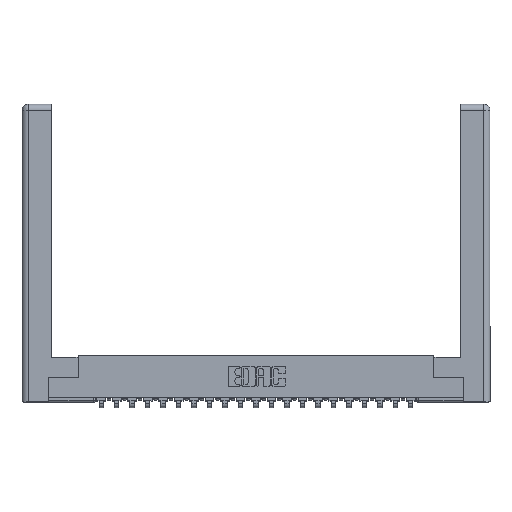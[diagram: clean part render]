
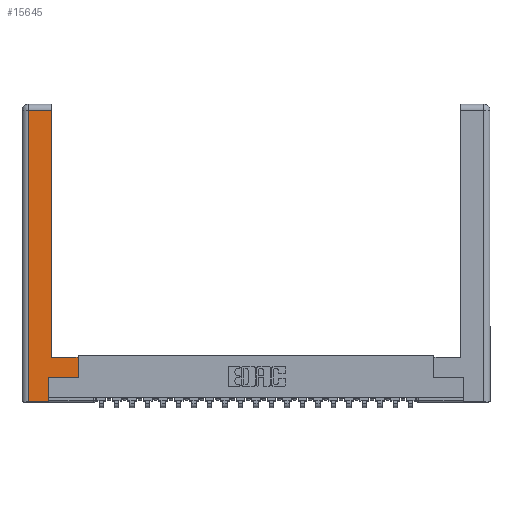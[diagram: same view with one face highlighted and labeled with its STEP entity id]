
A CAD part, top view. The second image highlights one B-rep face of the part: STEP entity #15645.
In plain terms, the highlighted planar face has unit normal (0, 0, 1).
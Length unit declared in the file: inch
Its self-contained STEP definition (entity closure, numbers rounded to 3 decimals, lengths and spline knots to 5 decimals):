
#306 = PLANE ( 'NONE',  #10145 ) ;
#809 = CARTESIAN_POINT ( 'NONE',  ( 0.295, 0.45, 0. ) ) ;
#877 = EDGE_CURVE ( 'NONE', #16083, #6153, #20618, .T. ) ;
#1115 = CARTESIAN_POINT ( 'NONE',  ( 0.265, 0., 0. ) ) ;
#1263 = ORIENTED_EDGE ( 'NONE', *, *, #13208, .T. ) ;
#1589 = VECTOR ( 'NONE', #19263, 39.37008 ) ;
#1649 = DIRECTION ( 'NONE',  ( 0., -1., 0. ) ) ;
#1656 = ORIENTED_EDGE ( 'NONE', *, *, #18970, .T. ) ;
#2031 = DIRECTION ( 'NONE',  ( -1., 0., 0. ) ) ;
#2057 = LINE ( 'NONE', #20446, #7541 ) ;
#2531 = ORIENTED_EDGE ( 'NONE', *, *, #13943, .T. ) ;
#2829 = LINE ( 'NONE', #1115, #1589 ) ;
#3650 = VERTEX_POINT ( 'NONE', #5099 ) ;
#3750 = ORIENTED_EDGE ( 'NONE', *, *, #877, .T. ) ;
#4056 = ORIENTED_EDGE ( 'NONE', *, *, #12929, .T. ) ;
#4154 = CARTESIAN_POINT ( 'NONE',  ( 0.265, 0.245, 0. ) ) ;
#5099 = CARTESIAN_POINT ( 'NONE',  ( 0.265, 0., 0. ) ) ;
#6027 = CARTESIAN_POINT ( 'NONE',  ( 0.565, 0.45, 0. ) ) ;
#6153 = VERTEX_POINT ( 'NONE', #6720 ) ;
#6720 = CARTESIAN_POINT ( 'NONE',  ( 0.295, 2.94, 0. ) ) ;
#7017 = ORIENTED_EDGE ( 'NONE', *, *, #14044, .T. ) ;
#7489 = VERTEX_POINT ( 'NONE', #21320 ) ;
#7541 = VECTOR ( 'NONE', #19099, 39.37008 ) ;
#8153 = VERTEX_POINT ( 'NONE', #20661 ) ;
#8188 = LINE ( 'NONE', #22556, #16856 ) ;
#8681 = VECTOR ( 'NONE', #20383, 39.37008 ) ;
#8954 = CARTESIAN_POINT ( 'NONE',  ( 0.0615, 0., 0. ) ) ;
#8990 = ORIENTED_EDGE ( 'NONE', *, *, #10652, .T. ) ;
#9011 = CARTESIAN_POINT ( 'NONE',  ( 0.0615, 0., 0. ) ) ;
#9062 = DIRECTION ( 'NONE',  ( 0., 1., 0. ) ) ;
#10145 = AXIS2_PLACEMENT_3D ( 'NONE', #20664, #11296, #2031 ) ;
#10652 = EDGE_CURVE ( 'NONE', #18060, #3650, #2829, .T. ) ;
#11296 = DIRECTION ( 'NONE',  ( 0., 0., -1. ) ) ;
#12262 = VERTEX_POINT ( 'NONE', #4154 ) ;
#12383 = ORIENTED_EDGE ( 'NONE', *, *, #21608, .T. ) ;
#12608 = VECTOR ( 'NONE', #20359, 39.37008 ) ;
#12929 = EDGE_CURVE ( 'NONE', #3650, #12262, #22329, .T. ) ;
#12940 = CARTESIAN_POINT ( 'NONE',  ( 0.565, 0.245, 0. ) ) ;
#13076 = CARTESIAN_POINT ( 'NONE',  ( 0.265, 0.245, 0. ) ) ;
#13208 = EDGE_CURVE ( 'NONE', #6153, #7489, #8188, .T. ) ;
#13326 = CARTESIAN_POINT ( 'NONE',  ( 0.295, 0.45, 0. ) ) ;
#13896 = VECTOR ( 'NONE', #9062, 39.37008 ) ;
#13943 = EDGE_CURVE ( 'NONE', #21923, #16083, #15541, .T. ) ;
#14044 = EDGE_CURVE ( 'NONE', #8153, #21923, #2057, .T. ) ;
#15541 = LINE ( 'NONE', #809, #17268 ) ;
#15616 = DIRECTION ( 'NONE',  ( -1., 0., 0. ) ) ;
#15645 = ADVANCED_FACE ( 'NONE', ( #22366 ), #306, .F. ) ;
#15664 = DIRECTION ( 'NONE',  ( -1., 0., 0. ) ) ;
#16083 = VERTEX_POINT ( 'NONE', #13326 ) ;
#16856 = VECTOR ( 'NONE', #15616, 39.37008 ) ;
#17268 = VECTOR ( 'NONE', #15664, 39.37008 ) ;
#17886 = EDGE_LOOP ( 'NONE', ( #3750, #1263, #12383, #8990, #4056, #1656, #7017, #2531 ) ) ;
#18060 = VERTEX_POINT ( 'NONE', #9011 ) ;
#18473 = VECTOR ( 'NONE', #1649, 39.37008 ) ;
#18970 = EDGE_CURVE ( 'NONE', #12262, #8153, #22068, .T. ) ;
#19099 = DIRECTION ( 'NONE',  ( 0., 1., 0. ) ) ;
#19263 = DIRECTION ( 'NONE',  ( 1., 0., 0. ) ) ;
#20038 = LINE ( 'NONE', #8954, #18473 ) ;
#20359 = DIRECTION ( 'NONE',  ( 1., 0., 0. ) ) ;
#20383 = DIRECTION ( 'NONE',  ( 0., 1., 0. ) ) ;
#20446 = CARTESIAN_POINT ( 'NONE',  ( 0.565, 0.45, 0. ) ) ;
#20618 = LINE ( 'NONE', #22554, #13896 ) ;
#20661 = CARTESIAN_POINT ( 'NONE',  ( 0.565, 0.245, 0. ) ) ;
#20664 = CARTESIAN_POINT ( 'NONE',  ( 0., 0., 0. ) ) ;
#21320 = CARTESIAN_POINT ( 'NONE',  ( 0.0615, 2.94, 0. ) ) ;
#21608 = EDGE_CURVE ( 'NONE', #7489, #18060, #20038, .T. ) ;
#21923 = VERTEX_POINT ( 'NONE', #6027 ) ;
#22068 = LINE ( 'NONE', #12940, #12608 ) ;
#22329 = LINE ( 'NONE', #13076, #8681 ) ;
#22366 = FACE_OUTER_BOUND ( 'NONE', #17886, .T. ) ;
#22554 = CARTESIAN_POINT ( 'NONE',  ( 0.295, 3., 0. ) ) ;
#22556 = CARTESIAN_POINT ( 'NONE',  ( 0.0615, 2.94, 0. ) ) ;
